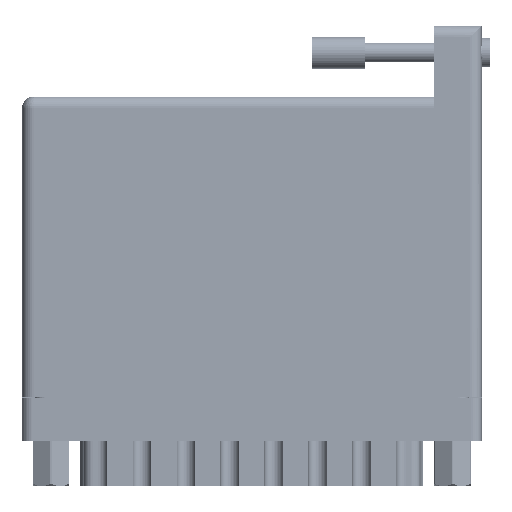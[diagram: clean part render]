
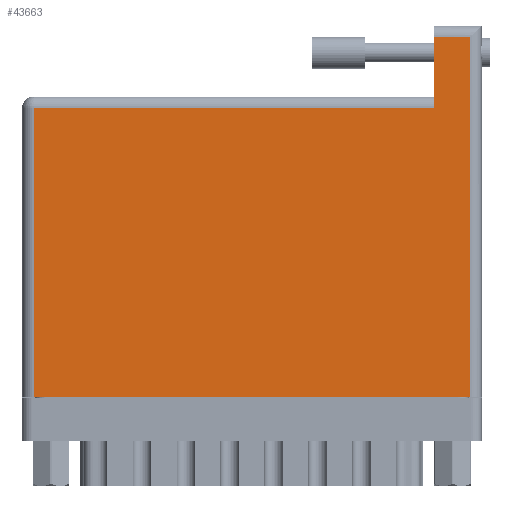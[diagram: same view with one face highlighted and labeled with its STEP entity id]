
A CAD part, front view. The second image highlights one B-rep face of the part: STEP entity #43663.
In plain terms, the highlighted face is planar.
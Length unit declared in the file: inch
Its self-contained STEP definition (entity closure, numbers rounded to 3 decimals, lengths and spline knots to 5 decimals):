
#2862 = EDGE_CURVE ( 'NONE', #27522, #19940, #13944, .T. ) ;
#5930 = DIRECTION ( 'NONE',  ( 1., 0., 0. ) ) ;
#6570 = EDGE_CURVE ( 'NONE', #69350, #74097, #80383, .T. ) ;
#8967 = LINE ( 'NONE', #81470, #69078 ) ;
#9711 = VECTOR ( 'NONE', #27613, 39.37008 ) ;
#9834 = CARTESIAN_POINT ( 'NONE',  ( 0., 2.125, 0. ) ) ;
#10358 = DIRECTION ( 'NONE',  ( -1., 0., 0. ) ) ;
#12253 = LINE ( 'NONE', #39583, #63055 ) ;
#13233 = EDGE_CURVE ( 'NONE', #46283, #27522, #58385, .T. ) ;
#13739 = DIRECTION ( 'NONE',  ( 0., -1., 0. ) ) ;
#13944 = LINE ( 'NONE', #84894, #64768 ) ;
#13993 = CARTESIAN_POINT ( 'NONE',  ( 2.438, 2.195, 0. ) ) ;
#15812 = CARTESIAN_POINT ( 'NONE',  ( 2.438, 2.125, 0. ) ) ;
#17048 = DIRECTION ( 'NONE',  ( -1., 0., 0. ) ) ;
#17783 = EDGE_CURVE ( 'NONE', #19940, #69350, #12253, .T. ) ;
#19429 = ORIENTED_EDGE ( 'NONE', *, *, #17783, .T. ) ;
#19940 = VERTEX_POINT ( 'NONE', #44960 ) ;
#25812 = DIRECTION ( 'NONE',  ( -1., 0., 0. ) ) ;
#27522 = VERTEX_POINT ( 'NONE', #48807 ) ;
#27613 = DIRECTION ( 'NONE',  ( 0., -1., 0. ) ) ;
#28911 = FACE_OUTER_BOUND ( 'NONE', #66482, .T. ) ;
#29307 = ORIENTED_EDGE ( 'NONE', *, *, #2862, .T. ) ;
#32388 = CARTESIAN_POINT ( 'NONE',  ( 0.07, 0., 0. ) ) ;
#33286 = CARTESIAN_POINT ( 'NONE',  ( 2.648, 2.125, 0. ) ) ;
#33661 = VERTEX_POINT ( 'NONE', #33286 ) ;
#39253 = EDGE_CURVE ( 'NONE', #33661, #46283, #74210, .T. ) ;
#39583 = CARTESIAN_POINT ( 'NONE',  ( 0.07, 0., 0. ) ) ;
#39961 = VECTOR ( 'NONE', #5930, 39.37008 ) ;
#39971 = ORIENTED_EDGE ( 'NONE', *, *, #39253, .T. ) ;
#41828 = DIRECTION ( 'NONE',  ( 0., 1., 0. ) ) ;
#42666 = AXIS2_PLACEMENT_3D ( 'NONE', #76389, #83032, #10358 ) ;
#43663 = ADVANCED_FACE ( 'NONE', ( #28911 ), #69793, .F. ) ;
#44960 = CARTESIAN_POINT ( 'NONE',  ( 0.07, 1.705, 0. ) ) ;
#46283 = VERTEX_POINT ( 'NONE', #15812 ) ;
#47256 = VECTOR ( 'NONE', #17048, 39.37008 ) ;
#48807 = CARTESIAN_POINT ( 'NONE',  ( 2.438, 1.705, 0. ) ) ;
#55448 = ORIENTED_EDGE ( 'NONE', *, *, #6570, .T. ) ;
#56707 = ORIENTED_EDGE ( 'NONE', *, *, #13233, .T. ) ;
#58385 = LINE ( 'NONE', #13993, #9711 ) ;
#58643 = EDGE_CURVE ( 'NONE', #74097, #33661, #8967, .T. ) ;
#63055 = VECTOR ( 'NONE', #13739, 39.37008 ) ;
#64768 = VECTOR ( 'NONE', #25812, 39.37008 ) ;
#65251 = CARTESIAN_POINT ( 'NONE',  ( 2.648, 0., 0. ) ) ;
#66482 = EDGE_LOOP ( 'NONE', ( #29307, #19429, #55448, #84880, #39971, #56707 ) ) ;
#69078 = VECTOR ( 'NONE', #41828, 39.37008 ) ;
#69350 = VERTEX_POINT ( 'NONE', #32388 ) ;
#69793 = PLANE ( 'NONE',  #42666 ) ;
#71974 = CARTESIAN_POINT ( 'NONE',  ( 0., 0., 0. ) ) ;
#74097 = VERTEX_POINT ( 'NONE', #65251 ) ;
#74210 = LINE ( 'NONE', #9834, #47256 ) ;
#76389 = CARTESIAN_POINT ( 'NONE',  ( 0., 1.775, 0. ) ) ;
#80383 = LINE ( 'NONE', #71974, #39961 ) ;
#81470 = CARTESIAN_POINT ( 'NONE',  ( 2.648, 2.195, 0. ) ) ;
#83032 = DIRECTION ( 'NONE',  ( 0., 0., -1. ) ) ;
#84880 = ORIENTED_EDGE ( 'NONE', *, *, #58643, .T. ) ;
#84894 = CARTESIAN_POINT ( 'NONE',  ( 0., 1.705, 0. ) ) ;
